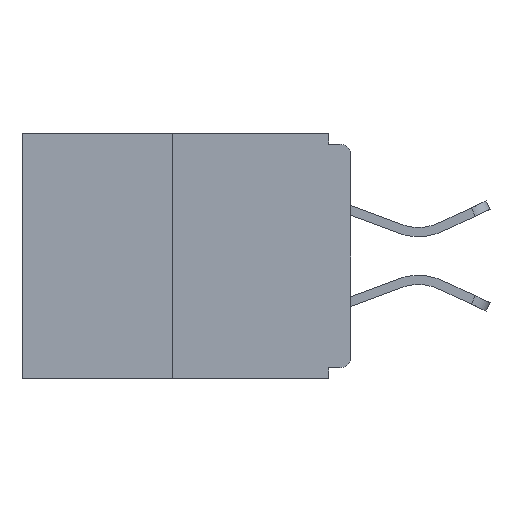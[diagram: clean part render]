
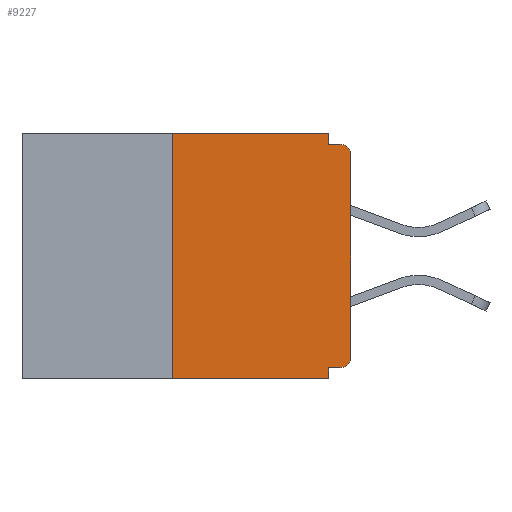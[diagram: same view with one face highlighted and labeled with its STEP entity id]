
A CAD part, left-side view. The second image highlights one B-rep face of the part: STEP entity #9227.
In plain terms, the highlighted planar face has unit normal (-1, 0, 0).
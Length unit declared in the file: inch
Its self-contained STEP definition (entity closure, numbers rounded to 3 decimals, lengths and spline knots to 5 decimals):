
#173 = AXIS2_PLACEMENT_3D ( 'NONE', #13263, #3987, #13365 ) ;
#306 = CARTESIAN_POINT ( 'NONE',  ( 0., 0.46, 0. ) ) ;
#647 = CARTESIAN_POINT ( 'NONE',  ( 0., 0.031, -0.343 ) ) ;
#984 = EDGE_CURVE ( 'NONE', #9396, #18286, #10176, .T. ) ;
#1107 = CARTESIAN_POINT ( 'NONE',  ( 0., 0.25, -0.343 ) ) ;
#1426 = CIRCLE ( 'NONE', #9894, 0.015 ) ;
#1527 = DIRECTION ( 'NONE',  ( 0., -1., 0. ) ) ;
#1835 = ORIENTED_EDGE ( 'NONE', *, *, #13908, .F. ) ;
#2284 = CARTESIAN_POINT ( 'NONE',  ( 0., 0.015, -0.015 ) ) ;
#2309 = VECTOR ( 'NONE', #15611, 39.37008 ) ;
#2335 = VERTEX_POINT ( 'NONE', #1107 ) ;
#2835 = ORIENTED_EDGE ( 'NONE', *, *, #984, .T. ) ;
#3573 = VERTEX_POINT ( 'NONE', #7370 ) ;
#3625 = VERTEX_POINT ( 'NONE', #17027 ) ;
#3637 = LINE ( 'NONE', #11254, #13902 ) ;
#3714 = DIRECTION ( 'NONE',  ( 0., 0., 1. ) ) ;
#3721 = LINE ( 'NONE', #22969, #17472 ) ;
#3927 = EDGE_CURVE ( 'NONE', #24478, #15316, #1426, .T. ) ;
#3987 = DIRECTION ( 'NONE',  ( 1., 0., 0. ) ) ;
#4558 = DIRECTION ( 'NONE',  ( 0., 0., -1. ) ) ;
#4934 = ORIENTED_EDGE ( 'NONE', *, *, #3927, .T. ) ;
#5364 = VECTOR ( 'NONE', #11306, 39.37008 ) ;
#5370 = LINE ( 'NONE', #17527, #2309 ) ;
#6503 = VECTOR ( 'NONE', #11912, 39.37008 ) ;
#6523 = VERTEX_POINT ( 'NONE', #7958 ) ;
#6786 = VERTEX_POINT ( 'NONE', #647 ) ;
#6816 = ORIENTED_EDGE ( 'NONE', *, *, #24260, .F. ) ;
#7370 = CARTESIAN_POINT ( 'NONE',  ( 0., 0.25, 0. ) ) ;
#7391 = VECTOR ( 'NONE', #1527, 39.37008 ) ;
#7545 = DIRECTION ( 'NONE',  ( 0., 0., 1. ) ) ;
#7754 = CARTESIAN_POINT ( 'NONE',  ( 0., 0., -0.03 ) ) ;
#7958 = CARTESIAN_POINT ( 'NONE',  ( 0., 0.031, -0.328 ) ) ;
#8132 = CARTESIAN_POINT ( 'NONE',  ( 0., 0., -0.328 ) ) ;
#8344 = EDGE_CURVE ( 'NONE', #2335, #6786, #17013, .T. ) ;
#8685 = VERTEX_POINT ( 'NONE', #18118 ) ;
#9227 = ADVANCED_FACE ( 'NONE', ( #11836 ), #21319, .F. ) ;
#9282 = DIRECTION ( 'NONE',  ( 0., 0., -1. ) ) ;
#9396 = VERTEX_POINT ( 'NONE', #22093 ) ;
#9448 = DIRECTION ( 'NONE',  ( -1., 0., 0. ) ) ;
#9547 = EDGE_CURVE ( 'NONE', #2335, #3573, #13336, .T. ) ;
#9894 = AXIS2_PLACEMENT_3D ( 'NONE', #12772, #9448, #16690 ) ;
#10176 = CIRCLE ( 'NONE', #15826, 0.015 ) ;
#10449 = EDGE_CURVE ( 'NONE', #9396, #6523, #18020, .T. ) ;
#11158 = LINE ( 'NONE', #18884, #7391 ) ;
#11254 = CARTESIAN_POINT ( 'NONE',  ( 0., 0., 0. ) ) ;
#11306 = DIRECTION ( 'NONE',  ( 0., -1., 0. ) ) ;
#11836 = FACE_OUTER_BOUND ( 'NONE', #20704, .T. ) ;
#11912 = DIRECTION ( 'NONE',  ( 0., -1., 0. ) ) ;
#12772 = CARTESIAN_POINT ( 'NONE',  ( 0., 0.015, -0.03 ) ) ;
#13263 = CARTESIAN_POINT ( 'NONE',  ( 0., 0.46, 0. ) ) ;
#13297 = ORIENTED_EDGE ( 'NONE', *, *, #21437, .F. ) ;
#13336 = LINE ( 'NONE', #21404, #16740 ) ;
#13365 = DIRECTION ( 'NONE',  ( 0., 0., -1. ) ) ;
#13902 = VECTOR ( 'NONE', #7545, 39.37008 ) ;
#13908 = EDGE_CURVE ( 'NONE', #3573, #3625, #18106, .T. ) ;
#15290 = EDGE_CURVE ( 'NONE', #8685, #15316, #11158, .T. ) ;
#15316 = VERTEX_POINT ( 'NONE', #2284 ) ;
#15491 = DIRECTION ( 'NONE',  ( 0., 1., 0. ) ) ;
#15611 = DIRECTION ( 'NONE',  ( 0., 0., -1. ) ) ;
#15826 = AXIS2_PLACEMENT_3D ( 'NONE', #18227, #23916, #4558 ) ;
#16051 = ORIENTED_EDGE ( 'NONE', *, *, #10449, .F. ) ;
#16690 = DIRECTION ( 'NONE',  ( 0., 0., -1. ) ) ;
#16740 = VECTOR ( 'NONE', #3714, 39.37008 ) ;
#16853 = EDGE_CURVE ( 'NONE', #18286, #24478, #3637, .T. ) ;
#17013 = LINE ( 'NONE', #21162, #5364 ) ;
#17027 = CARTESIAN_POINT ( 'NONE',  ( 0., 0.031, 0. ) ) ;
#17472 = VECTOR ( 'NONE', #9282, 39.37008 ) ;
#17527 = CARTESIAN_POINT ( 'NONE',  ( 0., 0.031, -0.343 ) ) ;
#18020 = LINE ( 'NONE', #8132, #23439 ) ;
#18106 = LINE ( 'NONE', #306, #6503 ) ;
#18118 = CARTESIAN_POINT ( 'NONE',  ( 0., 0.031, -0.015 ) ) ;
#18227 = CARTESIAN_POINT ( 'NONE',  ( 0., 0.015, -0.313 ) ) ;
#18286 = VERTEX_POINT ( 'NONE', #20676 ) ;
#18884 = CARTESIAN_POINT ( 'NONE',  ( 0., 0., -0.015 ) ) ;
#19403 = ORIENTED_EDGE ( 'NONE', *, *, #9547, .F. ) ;
#19868 = ORIENTED_EDGE ( 'NONE', *, *, #8344, .T. ) ;
#20676 = CARTESIAN_POINT ( 'NONE',  ( 0., 0., -0.313 ) ) ;
#20704 = EDGE_LOOP ( 'NONE', ( #1835, #19403, #19868, #13297, #16051, #2835, #22154, #4934, #23787, #6816 ) ) ;
#21162 = CARTESIAN_POINT ( 'NONE',  ( 0., 0.46, -0.343 ) ) ;
#21319 = PLANE ( 'NONE',  #173 ) ;
#21404 = CARTESIAN_POINT ( 'NONE',  ( 0., 0.25, 0. ) ) ;
#21437 = EDGE_CURVE ( 'NONE', #6523, #6786, #5370, .T. ) ;
#22093 = CARTESIAN_POINT ( 'NONE',  ( 0., 0.015, -0.328 ) ) ;
#22154 = ORIENTED_EDGE ( 'NONE', *, *, #16853, .T. ) ;
#22969 = CARTESIAN_POINT ( 'NONE',  ( 0., 0.031, 0. ) ) ;
#23439 = VECTOR ( 'NONE', #15491, 39.37008 ) ;
#23787 = ORIENTED_EDGE ( 'NONE', *, *, #15290, .F. ) ;
#23916 = DIRECTION ( 'NONE',  ( -1., 0., 0. ) ) ;
#24260 = EDGE_CURVE ( 'NONE', #3625, #8685, #3721, .T. ) ;
#24478 = VERTEX_POINT ( 'NONE', #7754 ) ;
